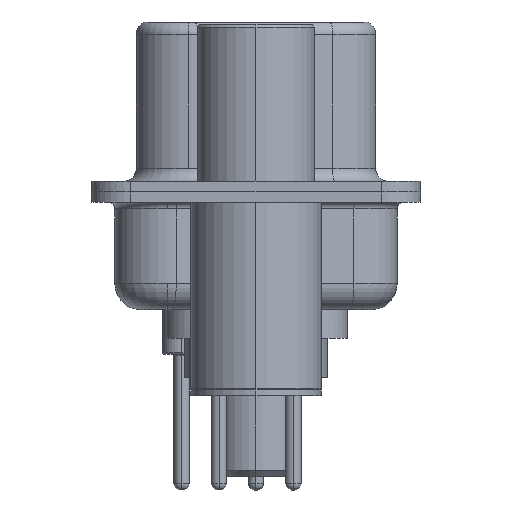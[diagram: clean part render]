
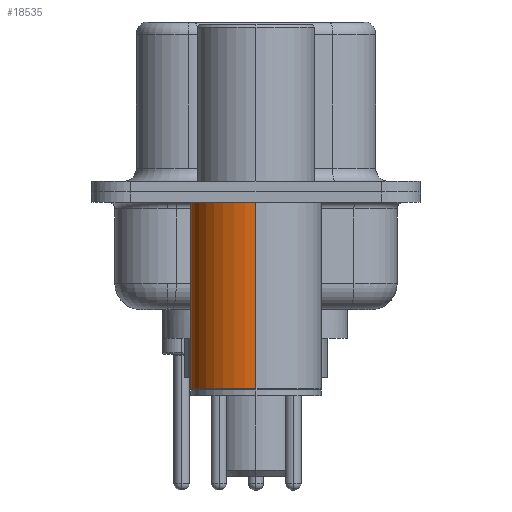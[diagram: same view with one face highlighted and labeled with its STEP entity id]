
A CAD part, left-side view. The second image highlights one B-rep face of the part: STEP entity #18535.
In plain terms, the highlighted cylindrical face has radius 2.5 mm (diameter 5 mm), a partial arc.
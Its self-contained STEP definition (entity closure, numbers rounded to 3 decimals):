
#37 = AXIS2_PLACEMENT_3D ( 'NONE', #10984, #17849, #9403 ) ;
#345 = ORIENTED_EDGE ( 'NONE', *, *, #22128, .T. ) ;
#1377 = CARTESIAN_POINT ( 'NONE',  ( -2.5, 0., 0.581 ) ) ;
#1518 = CARTESIAN_POINT ( 'NONE',  ( -2.5, 0., -7.525 ) ) ;
#2212 = LINE ( 'NONE', #3910, #17681 ) ;
#2436 = VERTEX_POINT ( 'NONE', #1518 ) ;
#3910 = CARTESIAN_POINT ( 'NONE',  ( 2.5, 0., 0.581 ) ) ;
#4484 = EDGE_CURVE ( 'NONE', #7685, #18191, #2212, .T. ) ;
#5930 = EDGE_CURVE ( 'NONE', #7685, #2436, #11468, .T. ) ;
#6251 = ORIENTED_EDGE ( 'NONE', *, *, #4484, .F. ) ;
#6666 = CYLINDRICAL_SURFACE ( 'NONE', #37, 2.5 ) ;
#7135 = ORIENTED_EDGE ( 'NONE', *, *, #19161, .F. ) ;
#7685 = VERTEX_POINT ( 'NONE', #18235 ) ;
#8269 = CARTESIAN_POINT ( 'NONE',  ( -2.5, 0., -0.4 ) ) ;
#9223 = CARTESIAN_POINT ( 'NONE',  ( 0., 0., -7.525 ) ) ;
#9403 = DIRECTION ( 'NONE',  ( 1., 0., 0. ) ) ;
#9462 = DIRECTION ( 'NONE',  ( 1., 0., 0. ) ) ;
#10984 = CARTESIAN_POINT ( 'NONE',  ( 0., 0., 0.581 ) ) ;
#11468 = CIRCLE ( 'NONE', #14463, 2.5 ) ;
#12382 = ORIENTED_EDGE ( 'NONE', *, *, #5930, .T. ) ;
#12556 = DIRECTION ( 'NONE',  ( 0., 0., 1. ) ) ;
#12883 = DIRECTION ( 'NONE',  ( 0., 0., 1. ) ) ;
#14103 = EDGE_LOOP ( 'NONE', ( #12382, #345, #7135, #6251 ) ) ;
#14238 = LINE ( 'NONE', #1377, #15844 ) ;
#14463 = AXIS2_PLACEMENT_3D ( 'NONE', #9223, #12556, #16040 ) ;
#14519 = DIRECTION ( 'NONE',  ( 0., 0., 1. ) ) ;
#15109 = FACE_OUTER_BOUND ( 'NONE', #14103, .T. ) ;
#15235 = DIRECTION ( 'NONE',  ( 0., 0., 1. ) ) ;
#15844 = VECTOR ( 'NONE', #15235, 1000. ) ;
#15904 = CARTESIAN_POINT ( 'NONE',  ( 2.5, 0., -0.4 ) ) ;
#16040 = DIRECTION ( 'NONE',  ( 1., 0., 0. ) ) ;
#16208 = CARTESIAN_POINT ( 'NONE',  ( 0., 0., -0.4 ) ) ;
#17681 = VECTOR ( 'NONE', #14519, 1000. ) ;
#17849 = DIRECTION ( 'NONE',  ( 0., 0., 1. ) ) ;
#18191 = VERTEX_POINT ( 'NONE', #15904 ) ;
#18235 = CARTESIAN_POINT ( 'NONE',  ( 2.5, 0., -7.525 ) ) ;
#18535 = ADVANCED_FACE ( 'NONE', ( #15109 ), #6666, .T. ) ;
#19161 = EDGE_CURVE ( 'NONE', #18191, #20193, #19696, .T. ) ;
#19696 = CIRCLE ( 'NONE', #20983, 2.5 ) ;
#20193 = VERTEX_POINT ( 'NONE', #8269 ) ;
#20983 = AXIS2_PLACEMENT_3D ( 'NONE', #16208, #12883, #9462 ) ;
#22128 = EDGE_CURVE ( 'NONE', #2436, #20193, #14238, .T. ) ;
